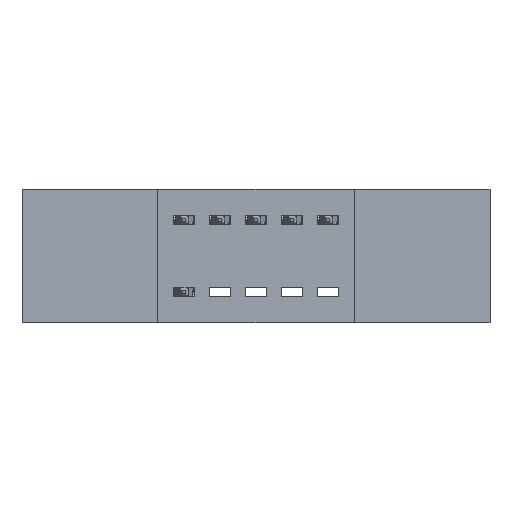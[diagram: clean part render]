
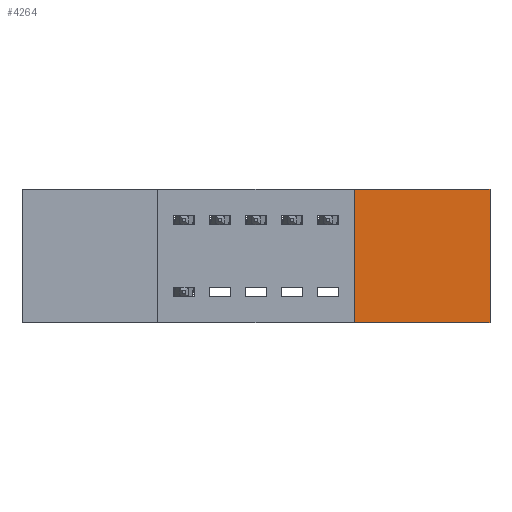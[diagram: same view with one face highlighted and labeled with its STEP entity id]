
A CAD part, front view. The second image highlights one B-rep face of the part: STEP entity #4264.
In plain terms, the highlighted planar face has unit normal (0, -1, 0).
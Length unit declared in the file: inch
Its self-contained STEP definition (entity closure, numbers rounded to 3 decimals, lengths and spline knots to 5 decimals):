
#101 = CARTESIAN_POINT ( 'NONE',  ( 1.3, 0., 0. ) ) ;
#200 = VECTOR ( 'NONE', #4104, 39.37008 ) ;
#548 = VERTEX_POINT ( 'NONE', #7206 ) ;
#633 = EDGE_CURVE ( 'NONE', #753, #849, #1626, .T. ) ;
#726 = CARTESIAN_POINT ( 'NONE',  ( 0.923, 0., -0.37 ) ) ;
#753 = VERTEX_POINT ( 'NONE', #101 ) ;
#849 = VERTEX_POINT ( 'NONE', #7083 ) ;
#927 = CARTESIAN_POINT ( 'NONE',  ( 0., 0., 0. ) ) ;
#1379 = PLANE ( 'NONE',  #4327 ) ;
#1455 = LINE ( 'NONE', #927, #2752 ) ;
#1626 = LINE ( 'NONE', #4622, #7578 ) ;
#1790 = ORIENTED_EDGE ( 'NONE', *, *, #6871, .F. ) ;
#2489 = DIRECTION ( 'NONE',  ( 0., 0., -1. ) ) ;
#2735 = CARTESIAN_POINT ( 'NONE',  ( 0., 0., -0.37 ) ) ;
#2752 = VECTOR ( 'NONE', #3459, 39.37008 ) ;
#2842 = ORIENTED_EDGE ( 'NONE', *, *, #633, .F. ) ;
#3046 = DIRECTION ( 'NONE',  ( 0., -1., 0. ) ) ;
#3122 = LINE ( 'NONE', #5477, #200 ) ;
#3145 = ORIENTED_EDGE ( 'NONE', *, *, #5089, .F. ) ;
#3459 = DIRECTION ( 'NONE',  ( 1., 0., 0. ) ) ;
#3648 = DIRECTION ( 'NONE',  ( -1., 0., 0. ) ) ;
#3900 = CARTESIAN_POINT ( 'NONE',  ( 0., 0., -0.37 ) ) ;
#4104 = DIRECTION ( 'NONE',  ( 0., 0., 1. ) ) ;
#4264 = ADVANCED_FACE ( 'NONE', ( #6516 ), #1379, .T. ) ;
#4327 = AXIS2_PLACEMENT_3D ( 'NONE', #2735, #3046, #2489 ) ;
#4378 = ORIENTED_EDGE ( 'NONE', *, *, #5168, .F. ) ;
#4622 = CARTESIAN_POINT ( 'NONE',  ( 1.3, 0., 0. ) ) ;
#5089 = EDGE_CURVE ( 'NONE', #7782, #548, #3122, .T. ) ;
#5168 = EDGE_CURVE ( 'NONE', #548, #753, #1455, .T. ) ;
#5477 = CARTESIAN_POINT ( 'NONE',  ( 0.923, 0., -0.37 ) ) ;
#5478 = VECTOR ( 'NONE', #3648, 39.37008 ) ;
#5688 = DIRECTION ( 'NONE',  ( 0., 0., -1. ) ) ;
#6516 = FACE_OUTER_BOUND ( 'NONE', #7301, .T. ) ;
#6871 = EDGE_CURVE ( 'NONE', #849, #7782, #7037, .T. ) ;
#7037 = LINE ( 'NONE', #3900, #5478 ) ;
#7083 = CARTESIAN_POINT ( 'NONE',  ( 1.3, 0., -0.37 ) ) ;
#7206 = CARTESIAN_POINT ( 'NONE',  ( 0.923, 0., 0. ) ) ;
#7301 = EDGE_LOOP ( 'NONE', ( #3145, #1790, #2842, #4378 ) ) ;
#7578 = VECTOR ( 'NONE', #5688, 39.37008 ) ;
#7782 = VERTEX_POINT ( 'NONE', #726 ) ;
